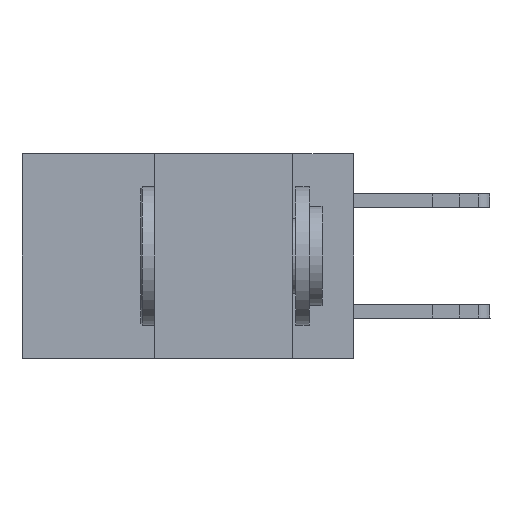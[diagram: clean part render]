
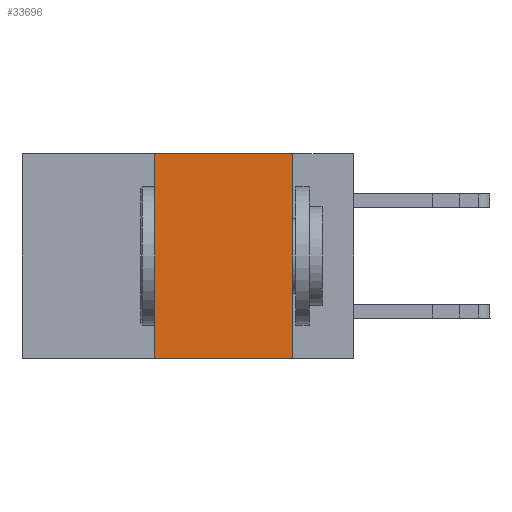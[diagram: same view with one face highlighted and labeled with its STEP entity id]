
A CAD part, left-side view. The second image highlights one B-rep face of the part: STEP entity #33696.
In plain terms, the highlighted planar face has unit normal (-1, 0, 0).
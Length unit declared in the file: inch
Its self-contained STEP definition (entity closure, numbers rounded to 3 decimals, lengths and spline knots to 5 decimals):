
#415 = DIRECTION ( 'NONE',  ( 0., 0., 1. ) ) ;
#811 = CARTESIAN_POINT ( 'NONE',  ( 0., 0.6, -0.37 ) ) ;
#3031 = EDGE_LOOP ( 'NONE', ( #7217, #31360, #33014, #25856 ) ) ;
#3311 = EDGE_CURVE ( 'NONE', #27928, #29588, #27632, .T. ) ;
#4568 = LINE ( 'NONE', #27974, #6260 ) ;
#5921 = CARTESIAN_POINT ( 'NONE',  ( 0., 0.11, 0. ) ) ;
#6260 = VECTOR ( 'NONE', #19813, 39.37008 ) ;
#6325 = AXIS2_PLACEMENT_3D ( 'NONE', #33412, #11901, #6360 ) ;
#6360 = DIRECTION ( 'NONE',  ( 0., 0., -1. ) ) ;
#6496 = FACE_OUTER_BOUND ( 'NONE', #3031, .T. ) ;
#7217 = ORIENTED_EDGE ( 'NONE', *, *, #14226, .F. ) ;
#7834 = VECTOR ( 'NONE', #415, 39.37008 ) ;
#8805 = VERTEX_POINT ( 'NONE', #5921 ) ;
#11804 = LINE ( 'NONE', #12381, #12664 ) ;
#11901 = DIRECTION ( 'NONE',  ( 1., 0., 0. ) ) ;
#12381 = CARTESIAN_POINT ( 'NONE',  ( 0., 0.6, 0. ) ) ;
#12664 = VECTOR ( 'NONE', #28980, 39.37008 ) ;
#13654 = CARTESIAN_POINT ( 'NONE',  ( 0., 0.36, 0. ) ) ;
#14226 = EDGE_CURVE ( 'NONE', #8805, #16472, #4568, .T. ) ;
#14994 = DIRECTION ( 'NONE',  ( 0., -1., 0. ) ) ;
#15178 = EDGE_CURVE ( 'NONE', #29588, #8805, #11804, .T. ) ;
#16472 = VERTEX_POINT ( 'NONE', #26639 ) ;
#17005 = CARTESIAN_POINT ( 'NONE',  ( 0., 0.36, -0.37 ) ) ;
#18743 = LINE ( 'NONE', #811, #27324 ) ;
#19813 = DIRECTION ( 'NONE',  ( 0., 0., -1. ) ) ;
#20032 = CARTESIAN_POINT ( 'NONE',  ( 0., 0.36, 0. ) ) ;
#25856 = ORIENTED_EDGE ( 'NONE', *, *, #30461, .T. ) ;
#26639 = CARTESIAN_POINT ( 'NONE',  ( 0., 0.11, -0.37 ) ) ;
#27324 = VECTOR ( 'NONE', #14994, 39.37008 ) ;
#27632 = LINE ( 'NONE', #20032, #7834 ) ;
#27928 = VERTEX_POINT ( 'NONE', #17005 ) ;
#27974 = CARTESIAN_POINT ( 'NONE',  ( 0., 0.11, 0. ) ) ;
#28980 = DIRECTION ( 'NONE',  ( 0., -1., 0. ) ) ;
#29588 = VERTEX_POINT ( 'NONE', #13654 ) ;
#30461 = EDGE_CURVE ( 'NONE', #27928, #16472, #18743, .T. ) ;
#30881 = PLANE ( 'NONE',  #6325 ) ;
#31360 = ORIENTED_EDGE ( 'NONE', *, *, #15178, .F. ) ;
#33014 = ORIENTED_EDGE ( 'NONE', *, *, #3311, .F. ) ;
#33412 = CARTESIAN_POINT ( 'NONE',  ( 0., 0.6, 0. ) ) ;
#33696 = ADVANCED_FACE ( 'NONE', ( #6496 ), #30881, .F. ) ;
